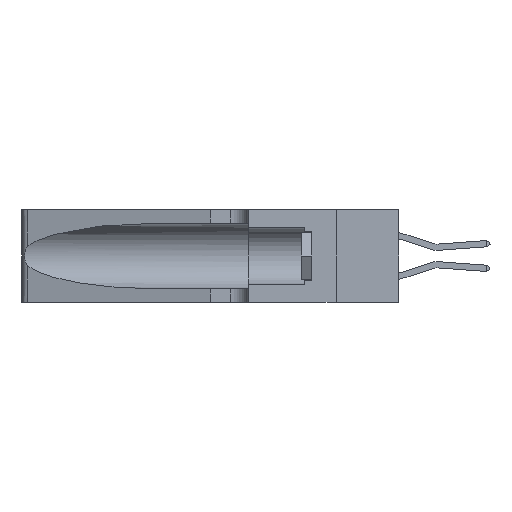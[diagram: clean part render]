
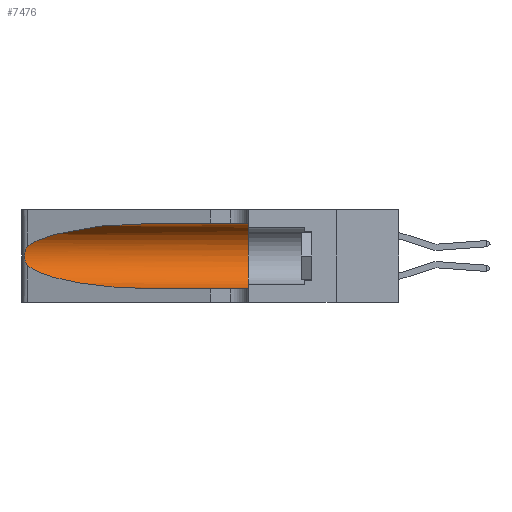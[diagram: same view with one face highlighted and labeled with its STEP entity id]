
A CAD part, left-side view. The second image highlights one B-rep face of the part: STEP entity #7476.
In plain terms, the highlighted cylindrical face has radius 3.308 mm (diameter 6.617 mm), a partial arc.
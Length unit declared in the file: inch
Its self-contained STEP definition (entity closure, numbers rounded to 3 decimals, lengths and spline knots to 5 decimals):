
#1202 = CARTESIAN_POINT ( 'NONE',  ( 0.1305, 1.61858, 0.185 ) ) ;
#1295 = CARTESIAN_POINT ( 'NONE',  ( 0.26075, 1.23896, 0.178 ) ) ;
#3076 = VECTOR ( 'NONE', #20503, 39.37008 ) ;
#4029 = DIRECTION ( 'NONE',  ( 0., 0., -1. ) ) ;
#4121 = CARTESIAN_POINT ( 'NONE',  ( 0.25856, 1.23593, 0.16098 ) ) ;
#5024 = EDGE_CURVE ( 'NONE', #16669, #24059, #19572, .T. ) ;
#5082 = EDGE_CURVE ( 'NONE', #24581, #16669, #17853, .T. ) ;
#5088 = CYLINDRICAL_SURFACE ( 'NONE', #12625, 0.13025 ) ;
#5457 = ORIENTED_EDGE ( 'NONE', *, *, #14655, .T. ) ;
#6428 = EDGE_CURVE ( 'NONE', #24581, #24069, #30669, .T. ) ;
#6829 = CARTESIAN_POINT ( 'NONE',  ( 0.25487, 1.22718, 0.22369 ) ) ;
#6948 = CARTESIAN_POINT ( 'NONE',  ( 0.25639, 1.23186, 0.15144 ) ) ;
#7079 = CARTESIAN_POINT ( 'NONE',  ( 0.1305, 0.72297, 0.05475 ) ) ;
#7476 = ADVANCED_FACE ( 'NONE', ( #27168 ), #5088, .F. ) ;
#8168 = VERTEX_POINT ( 'NONE', #15278 ) ;
#8742 = B_SPLINE_CURVE_WITH_KNOTS ( 'NONE', 3,
 ( #6829, #28792, #12422, #31720, #15185, #34487, #17960, #1295, #20730, #4121, #23501, #6948, #26280, #9753 ),
 .UNSPECIFIED., .F., .F.,
 ( 4, 2, 2, 2, 2, 2, 4 ),
 ( 0., 0.00027, 0.00053, 0.00107, 0.0016, 0.00187, 0.00214 ),
 .UNSPECIFIED. ) ;
#9272 = DIRECTION ( 'NONE',  ( 0., 1., 0. ) ) ;
#9753 = CARTESIAN_POINT ( 'NONE',  ( 0.25487, 1.22718, 0.14631 ) ) ;
#11735 = CARTESIAN_POINT ( 'NONE',  ( 0.1305, 0.72297, 0.31525 ) ) ;
#12422 = CARTESIAN_POINT ( 'NONE',  ( 0.25639, 1.23184, 0.21858 ) ) ;
#12625 = AXIS2_PLACEMENT_3D ( 'NONE', #1202, #20634, #4029 ) ;
#14629 = CARTESIAN_POINT ( 'NONE',  ( 0.1305, 1.61858, 0.05475 ) ) ;
#14655 = EDGE_CURVE ( 'NONE', #8168, #15489, #34439, .T. ) ;
#15185 = CARTESIAN_POINT ( 'NONE',  ( 0.25854, 1.2359, 0.20912 ) ) ;
#15278 = CARTESIAN_POINT ( 'NONE',  ( 0.25487, 1.22718, 0.14631 ) ) ;
#15489 = VERTEX_POINT ( 'NONE', #34089 ) ;
#16669 = VERTEX_POINT ( 'NONE', #17251 ) ;
#17240 = ORIENTED_EDGE ( 'NONE', *, *, #18054, .T. ) ;
#17251 = CARTESIAN_POINT ( 'NONE',  ( 0.1305, 0.35, 0.31525 ) ) ;
#17401 = DIRECTION ( 'NONE',  ( 0., -1., 0. ) ) ;
#17515 = EDGE_LOOP ( 'NONE', ( #34318, #24648, #5457, #17240, #18847, #29013 ) ) ;
#17733 = CARTESIAN_POINT ( 'NONE',  ( 0.1305, 1.61858, 0.31525 ) ) ;
#17853 = LINE ( 'NONE', #17733, #3076 ) ;
#17960 = CARTESIAN_POINT ( 'NONE',  ( 0.26075, 1.23896, 0.19203 ) ) ;
#18054 = EDGE_CURVE ( 'NONE', #15489, #24059, #25994, .T. ) ;
#18847 = ORIENTED_EDGE ( 'NONE', *, *, #5024, .F. ) ;
#19572 = CIRCLE ( 'NONE', #32893, 0.13025 ) ;
#20503 = DIRECTION ( 'NONE',  ( 0., -1., 0. ) ) ;
#20634 = DIRECTION ( 'NONE',  ( 0., -1., 0. ) ) ;
#20730 = CARTESIAN_POINT ( 'NONE',  ( 0.26017, 1.23833, 0.17102 ) ) ;
#20857 = CARTESIAN_POINT ( 'NONE',  ( 0.25487, 1.22718, 0.14631 ) ) ;
#22013 = CARTESIAN_POINT ( 'NONE',  ( 0.1305, 0.72297, 0.31525 ) ) ;
#23041 = EDGE_CURVE ( 'NONE', #24069, #8168, #8742, .T. ) ;
#23501 = CARTESIAN_POINT ( 'NONE',  ( 0.25789, 1.23486, 0.15765 ) ) ;
#23627 = CARTESIAN_POINT ( 'NONE',  ( 0.18966, 0.96281, 0.05475 ) ) ;
#24059 = VERTEX_POINT ( 'NONE', #35849 ) ;
#24069 = VERTEX_POINT ( 'NONE', #33216 ) ;
#24581 = VERTEX_POINT ( 'NONE', #11735 ) ;
#24648 = ORIENTED_EDGE ( 'NONE', *, *, #23041, .T. ) ;
#24800 = CARTESIAN_POINT ( 'NONE',  ( 0.18966, 0.96281, 0.31525 ) ) ;
#25816 = CARTESIAN_POINT ( 'NONE',  ( 0.1305, 0.35, 0.185 ) ) ;
#25994 = LINE ( 'NONE', #14629, #32463 ) ;
#26280 = CARTESIAN_POINT ( 'NONE',  ( 0.25555, 1.22993, 0.14849 ) ) ;
#27168 = FACE_OUTER_BOUND ( 'NONE', #17515, .T. ) ;
#27563 = CARTESIAN_POINT ( 'NONE',  ( 0.25487, 1.22718, 0.22369 ) ) ;
#28569 = DIRECTION ( 'NONE',  ( 0., 0., 1. ) ) ;
#28792 = CARTESIAN_POINT ( 'NONE',  ( 0.25555, 1.22994, 0.2215 ) ) ;
#29013 = ORIENTED_EDGE ( 'NONE', *, *, #5082, .F. ) ;
#30669 =( BOUNDED_CURVE ( )  B_SPLINE_CURVE ( 3, ( #22013, #24800, #33010, #27563 ),
 .UNSPECIFIED., .F., .F. ) 
 B_SPLINE_CURVE_WITH_KNOTS ( ( 4, 4 ),
 ( 1.5708, 2.84003 ),
 .UNSPECIFIED. ) 
 CURVE ( )  GEOMETRIC_REPRESENTATION_ITEM ( )  RATIONAL_B_SPLINE_CURVE ( ( 1., 0.87, 0.87, 1. ) ) 
 REPRESENTATION_ITEM ( '' )  );
#31720 = CARTESIAN_POINT ( 'NONE',  ( 0.25787, 1.23484, 0.2124 ) ) ;
#32463 = VECTOR ( 'NONE', #17401, 39.37008 ) ;
#32893 = AXIS2_PLACEMENT_3D ( 'NONE', #25816, #9272, #28569 ) ;
#33010 = CARTESIAN_POINT ( 'NONE',  ( 0.2373, 1.15595, 0.28018 ) ) ;
#33216 = CARTESIAN_POINT ( 'NONE',  ( 0.25487, 1.22718, 0.22369 ) ) ;
#34089 = CARTESIAN_POINT ( 'NONE',  ( 0.1305, 0.72297, 0.05475 ) ) ;
#34318 = ORIENTED_EDGE ( 'NONE', *, *, #6428, .T. ) ;
#34439 =( BOUNDED_CURVE ( )  B_SPLINE_CURVE ( 3, ( #20857, #34612, #23627, #7079 ),
 .UNSPECIFIED., .F., .F. ) 
 B_SPLINE_CURVE_WITH_KNOTS ( ( 4, 4 ),
 ( 3.44316, 4.71239 ),
 .UNSPECIFIED. ) 
 CURVE ( )  GEOMETRIC_REPRESENTATION_ITEM ( )  RATIONAL_B_SPLINE_CURVE ( ( 1., 0.87, 0.87, 1. ) ) 
 REPRESENTATION_ITEM ( '' )  );
#34487 = CARTESIAN_POINT ( 'NONE',  ( 0.26018, 1.23835, 0.19895 ) ) ;
#34612 = CARTESIAN_POINT ( 'NONE',  ( 0.2373, 1.15595, 0.08982 ) ) ;
#35849 = CARTESIAN_POINT ( 'NONE',  ( 0.1305, 0.35, 0.05475 ) ) ;
